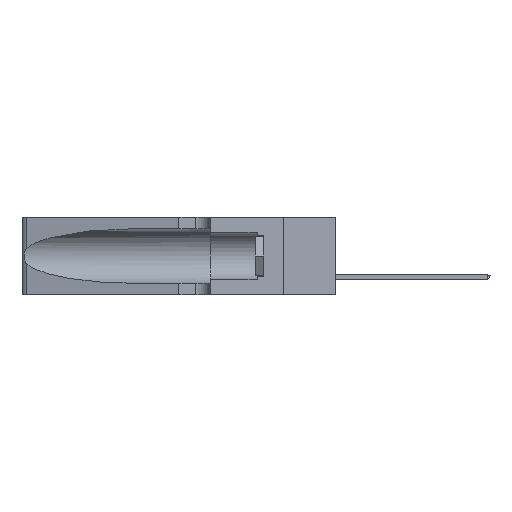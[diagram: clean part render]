
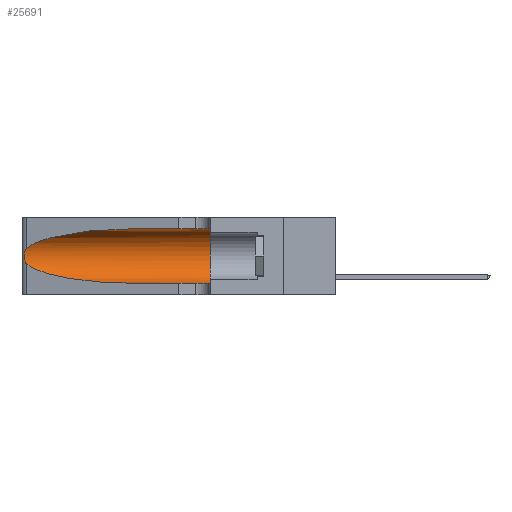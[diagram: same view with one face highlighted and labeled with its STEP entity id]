
A CAD part, left-side view. The second image highlights one B-rep face of the part: STEP entity #25691.
In plain terms, the highlighted cylindrical face has radius 3.308 mm (diameter 6.617 mm), a partial arc.
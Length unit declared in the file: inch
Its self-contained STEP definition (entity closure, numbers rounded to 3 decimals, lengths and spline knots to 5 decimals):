
#572 = CARTESIAN_POINT ( 'NONE',  ( 0.1305, 0.72297, 0.05475 ) ) ;
#1547 = EDGE_CURVE ( 'NONE', #15177, #16043, #9503, .T. ) ;
#2529 = AXIS2_PLACEMENT_3D ( 'NONE', #4244, #19127, #29159 ) ;
#2533 = CARTESIAN_POINT ( 'NONE',  ( 0.26017, 1.23833, 0.17102 ) ) ;
#3257 = CARTESIAN_POINT ( 'NONE',  ( 0.25487, 1.22718, 0.22369 ) ) ;
#3401 = CARTESIAN_POINT ( 'NONE',  ( 0.1305, 0.72297, 0.31525 ) ) ;
#3516 = CARTESIAN_POINT ( 'NONE',  ( 0.18966, 0.96281, 0.31525 ) ) ;
#3916 = ORIENTED_EDGE ( 'NONE', *, *, #20953, .T. ) ;
#4244 = CARTESIAN_POINT ( 'NONE',  ( 0.1305, 0.35, 0.185 ) ) ;
#4904 = CARTESIAN_POINT ( 'NONE',  ( 0.26075, 1.23896, 0.19203 ) ) ;
#5476 = VECTOR ( 'NONE', #27959, 39.37008 ) ;
#5802 = EDGE_CURVE ( 'NONE', #16043, #13533, #18690, .T. ) ;
#6655 = CARTESIAN_POINT ( 'NONE',  ( 0.25555, 1.22994, 0.2215 ) ) ;
#7067 = VERTEX_POINT ( 'NONE', #20098 ) ;
#7840 = CARTESIAN_POINT ( 'NONE',  ( 0.25789, 1.23486, 0.15765 ) ) ;
#8011 = LINE ( 'NONE', #27728, #17091 ) ;
#8077 = EDGE_LOOP ( 'NONE', ( #30741, #16467, #21220, #3916, #16605, #12414 ) ) ;
#9503 = B_SPLINE_CURVE_WITH_KNOTS ( 'NONE', 3,
 ( #3257, #6655, #13070, #17208, #25115, #27261, #4904, #9971, #2533, #15127, #7840, #15638, #23157, #15420 ),
 .UNSPECIFIED., .F., .F.,
 ( 4, 2, 2, 2, 2, 2, 4 ),
 ( 0., 0.00027, 0.00053, 0.00107, 0.0016, 0.00187, 0.00214 ),
 .UNSPECIFIED. ) ;
#9953 = DIRECTION ( 'NONE',  ( 0., -1., 0. ) ) ;
#9971 = CARTESIAN_POINT ( 'NONE',  ( 0.26075, 1.23896, 0.178 ) ) ;
#12414 = ORIENTED_EDGE ( 'NONE', *, *, #24047, .F. ) ;
#13070 = CARTESIAN_POINT ( 'NONE',  ( 0.25639, 1.23184, 0.21858 ) ) ;
#13478 = CARTESIAN_POINT ( 'NONE',  ( 0.1305, 1.61858, 0.185 ) ) ;
#13533 = VERTEX_POINT ( 'NONE', #572 ) ;
#14840 = EDGE_CURVE ( 'NONE', #7067, #15177, #27855, .T. ) ;
#14957 = CIRCLE ( 'NONE', #2529, 0.13025 ) ;
#15127 = CARTESIAN_POINT ( 'NONE',  ( 0.25856, 1.23593, 0.16098 ) ) ;
#15177 = VERTEX_POINT ( 'NONE', #20489 ) ;
#15420 = CARTESIAN_POINT ( 'NONE',  ( 0.25487, 1.22718, 0.14631 ) ) ;
#15638 = CARTESIAN_POINT ( 'NONE',  ( 0.25639, 1.23186, 0.15144 ) ) ;
#15725 = LINE ( 'NONE', #30330, #5476 ) ;
#16043 = VERTEX_POINT ( 'NONE', #19075 ) ;
#16168 = CARTESIAN_POINT ( 'NONE',  ( 0.25487, 1.22718, 0.14631 ) ) ;
#16467 = ORIENTED_EDGE ( 'NONE', *, *, #1547, .T. ) ;
#16605 = ORIENTED_EDGE ( 'NONE', *, *, #23600, .F. ) ;
#17091 = VECTOR ( 'NONE', #9953, 39.37008 ) ;
#17208 = CARTESIAN_POINT ( 'NONE',  ( 0.25787, 1.23484, 0.2124 ) ) ;
#17248 = AXIS2_PLACEMENT_3D ( 'NONE', #13478, #30906, #18063 ) ;
#18021 = CARTESIAN_POINT ( 'NONE',  ( 0.1305, 0.35, 0.05475 ) ) ;
#18063 = DIRECTION ( 'NONE',  ( 0., 0., -1. ) ) ;
#18332 = CARTESIAN_POINT ( 'NONE',  ( 0.1305, 0.72297, 0.05475 ) ) ;
#18690 =( BOUNDED_CURVE ( )  B_SPLINE_CURVE ( 3, ( #16168, #21041, #25852, #18332 ),
 .UNSPECIFIED., .F., .F. ) 
 B_SPLINE_CURVE_WITH_KNOTS ( ( 4, 4 ),
 ( 3.44316, 4.71239 ),
 .UNSPECIFIED. ) 
 CURVE ( )  GEOMETRIC_REPRESENTATION_ITEM ( )  RATIONAL_B_SPLINE_CURVE ( ( 1., 0.87, 0.87, 1. ) ) 
 REPRESENTATION_ITEM ( '' )  );
#18824 = CARTESIAN_POINT ( 'NONE',  ( 0.1305, 0.35, 0.31525 ) ) ;
#19075 = CARTESIAN_POINT ( 'NONE',  ( 0.25487, 1.22718, 0.14631 ) ) ;
#19127 = DIRECTION ( 'NONE',  ( 0., 1., 0. ) ) ;
#20098 = CARTESIAN_POINT ( 'NONE',  ( 0.1305, 0.72297, 0.31525 ) ) ;
#20489 = CARTESIAN_POINT ( 'NONE',  ( 0.25487, 1.22718, 0.22369 ) ) ;
#20541 = CARTESIAN_POINT ( 'NONE',  ( 0.2373, 1.15595, 0.28018 ) ) ;
#20953 = EDGE_CURVE ( 'NONE', #13533, #23431, #8011, .T. ) ;
#21041 = CARTESIAN_POINT ( 'NONE',  ( 0.2373, 1.15595, 0.08982 ) ) ;
#21220 = ORIENTED_EDGE ( 'NONE', *, *, #5802, .T. ) ;
#21733 = CYLINDRICAL_SURFACE ( 'NONE', #17248, 0.13025 ) ;
#23067 = CARTESIAN_POINT ( 'NONE',  ( 0.25487, 1.22718, 0.22369 ) ) ;
#23157 = CARTESIAN_POINT ( 'NONE',  ( 0.25555, 1.22993, 0.14849 ) ) ;
#23431 = VERTEX_POINT ( 'NONE', #18021 ) ;
#23600 = EDGE_CURVE ( 'NONE', #31155, #23431, #14957, .T. ) ;
#24047 = EDGE_CURVE ( 'NONE', #7067, #31155, #15725, .T. ) ;
#25115 = CARTESIAN_POINT ( 'NONE',  ( 0.25854, 1.2359, 0.20912 ) ) ;
#25691 = ADVANCED_FACE ( 'NONE', ( #28333 ), #21733, .F. ) ;
#25852 = CARTESIAN_POINT ( 'NONE',  ( 0.18966, 0.96281, 0.05475 ) ) ;
#27261 = CARTESIAN_POINT ( 'NONE',  ( 0.26018, 1.23835, 0.19895 ) ) ;
#27728 = CARTESIAN_POINT ( 'NONE',  ( 0.1305, 1.61858, 0.05475 ) ) ;
#27855 =( BOUNDED_CURVE ( )  B_SPLINE_CURVE ( 3, ( #3401, #3516, #20541, #23067 ),
 .UNSPECIFIED., .F., .F. ) 
 B_SPLINE_CURVE_WITH_KNOTS ( ( 4, 4 ),
 ( 1.5708, 2.84003 ),
 .UNSPECIFIED. ) 
 CURVE ( )  GEOMETRIC_REPRESENTATION_ITEM ( )  RATIONAL_B_SPLINE_CURVE ( ( 1., 0.87, 0.87, 1. ) ) 
 REPRESENTATION_ITEM ( '' )  );
#27959 = DIRECTION ( 'NONE',  ( 0., -1., 0. ) ) ;
#28333 = FACE_OUTER_BOUND ( 'NONE', #8077, .T. ) ;
#29159 = DIRECTION ( 'NONE',  ( 0., 0., 1. ) ) ;
#30330 = CARTESIAN_POINT ( 'NONE',  ( 0.1305, 1.61858, 0.31525 ) ) ;
#30741 = ORIENTED_EDGE ( 'NONE', *, *, #14840, .T. ) ;
#30906 = DIRECTION ( 'NONE',  ( 0., -1., 0. ) ) ;
#31155 = VERTEX_POINT ( 'NONE', #18824 ) ;
